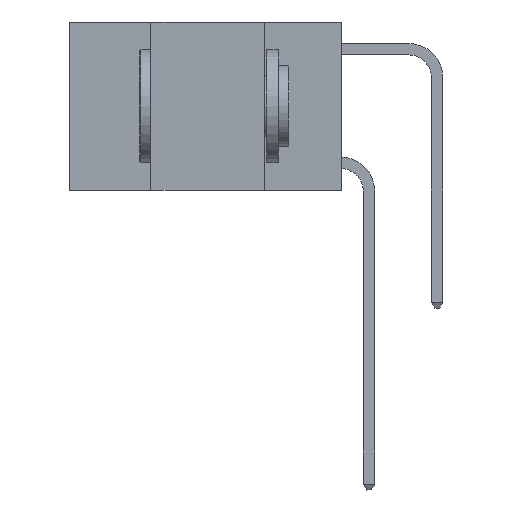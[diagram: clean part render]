
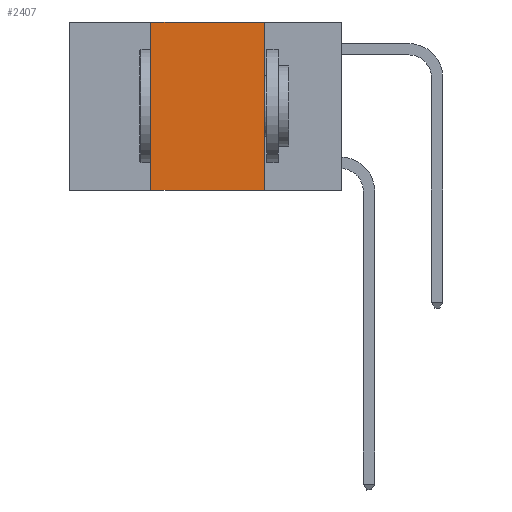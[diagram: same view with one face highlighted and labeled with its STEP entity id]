
A CAD part, left-side view. The second image highlights one B-rep face of the part: STEP entity #2407.
In plain terms, the highlighted planar face has unit normal (-1, 0, 0).
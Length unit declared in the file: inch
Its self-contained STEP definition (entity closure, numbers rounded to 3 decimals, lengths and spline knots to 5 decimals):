
#230 = DIRECTION ( 'NONE',  ( 0., 0., 1. ) ) ;
#368 = CARTESIAN_POINT ( 'NONE',  ( 0., 0.17, -0.37 ) ) ;
#788 = VERTEX_POINT ( 'NONE', #368 ) ;
#838 = CARTESIAN_POINT ( 'NONE',  ( 0., 0.6, 0. ) ) ;
#2290 = PLANE ( 'NONE',  #8233 ) ;
#2407 = ADVANCED_FACE ( 'NONE', ( #18277 ), #2290, .F. ) ;
#3312 = CARTESIAN_POINT ( 'NONE',  ( 0., 0.42, 0. ) ) ;
#3904 = CARTESIAN_POINT ( 'NONE',  ( 0., 0.6, -0.37 ) ) ;
#4078 = EDGE_CURVE ( 'NONE', #8372, #788, #4763, .T. ) ;
#4763 = LINE ( 'NONE', #6306, #6948 ) ;
#5802 = EDGE_CURVE ( 'NONE', #16090, #788, #12962, .T. ) ;
#5935 = LINE ( 'NONE', #6412, #6761 ) ;
#6306 = CARTESIAN_POINT ( 'NONE',  ( 0., 0.17, 0. ) ) ;
#6412 = CARTESIAN_POINT ( 'NONE',  ( 0., 0.6, 0. ) ) ;
#6526 = VERTEX_POINT ( 'NONE', #11154 ) ;
#6589 = CARTESIAN_POINT ( 'NONE',  ( 0., 0.17, 0. ) ) ;
#6761 = VECTOR ( 'NONE', #9499, 39.37008 ) ;
#6948 = VECTOR ( 'NONE', #12178, 39.37008 ) ;
#8233 = AXIS2_PLACEMENT_3D ( 'NONE', #838, #18469, #15544 ) ;
#8316 = EDGE_CURVE ( 'NONE', #6526, #8372, #5935, .T. ) ;
#8372 = VERTEX_POINT ( 'NONE', #6589 ) ;
#8502 = ORIENTED_EDGE ( 'NONE', *, *, #13102, .F. ) ;
#8989 = LINE ( 'NONE', #3312, #13021 ) ;
#9499 = DIRECTION ( 'NONE',  ( 0., -1., 0. ) ) ;
#9955 = ORIENTED_EDGE ( 'NONE', *, *, #5802, .T. ) ;
#11127 = DIRECTION ( 'NONE',  ( 0., -1., 0. ) ) ;
#11154 = CARTESIAN_POINT ( 'NONE',  ( 0., 0.42, 0. ) ) ;
#11574 = EDGE_LOOP ( 'NONE', ( #14144, #16753, #8502, #9955 ) ) ;
#12178 = DIRECTION ( 'NONE',  ( 0., 0., -1. ) ) ;
#12962 = LINE ( 'NONE', #3904, #13770 ) ;
#13021 = VECTOR ( 'NONE', #230, 39.37008 ) ;
#13102 = EDGE_CURVE ( 'NONE', #16090, #6526, #8989, .T. ) ;
#13299 = CARTESIAN_POINT ( 'NONE',  ( 0., 0.42, -0.37 ) ) ;
#13770 = VECTOR ( 'NONE', #11127, 39.37008 ) ;
#14144 = ORIENTED_EDGE ( 'NONE', *, *, #4078, .F. ) ;
#15544 = DIRECTION ( 'NONE',  ( 0., 0., -1. ) ) ;
#16090 = VERTEX_POINT ( 'NONE', #13299 ) ;
#16753 = ORIENTED_EDGE ( 'NONE', *, *, #8316, .F. ) ;
#18277 = FACE_OUTER_BOUND ( 'NONE', #11574, .T. ) ;
#18469 = DIRECTION ( 'NONE',  ( 1., 0., 0. ) ) ;
